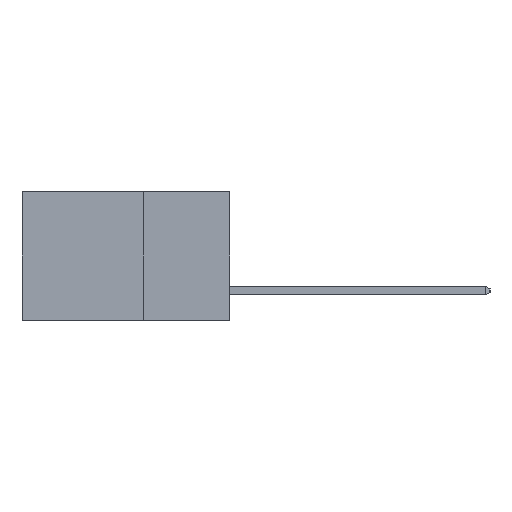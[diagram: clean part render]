
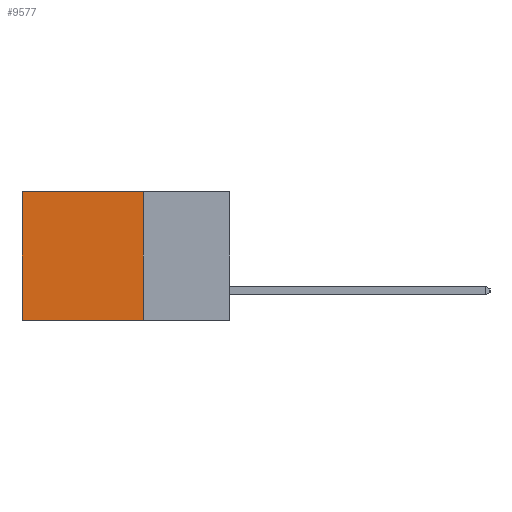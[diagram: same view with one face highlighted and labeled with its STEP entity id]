
A CAD part, left-side view. The second image highlights one B-rep face of the part: STEP entity #9577.
In plain terms, the highlighted planar face has unit normal (-1, 0, 0).
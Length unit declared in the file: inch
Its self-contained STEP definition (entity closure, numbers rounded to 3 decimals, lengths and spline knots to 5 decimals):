
#45 = ORIENTED_EDGE ( 'NONE', *, *, #4189, .F. ) ;
#303 = CARTESIAN_POINT ( 'NONE',  ( 0.298, 0.25, 0. ) ) ;
#1175 = LINE ( 'NONE', #14276, #4788 ) ;
#3883 = AXIS2_PLACEMENT_3D ( 'NONE', #303, #17476, #8109 ) ;
#4189 = EDGE_CURVE ( 'NONE', #13730, #6441, #7310, .T. ) ;
#4197 = ORIENTED_EDGE ( 'NONE', *, *, #18765, .T. ) ;
#4788 = VECTOR ( 'NONE', #6432, 39.37008 ) ;
#4801 = DIRECTION ( 'NONE',  ( 0., 0., -1. ) ) ;
#5476 = VERTEX_POINT ( 'NONE', #19278 ) ;
#5900 = CARTESIAN_POINT ( 'NONE',  ( 0.298, 0.25, -0.37 ) ) ;
#6020 = CARTESIAN_POINT ( 'NONE',  ( 0.298, 0.25, -0.37 ) ) ;
#6432 = DIRECTION ( 'NONE',  ( 0., 1., 0. ) ) ;
#6441 = VERTEX_POINT ( 'NONE', #9092 ) ;
#6531 = PLANE ( 'NONE',  #3883 ) ;
#7228 = VECTOR ( 'NONE', #4801, 39.37008 ) ;
#7310 = LINE ( 'NONE', #6020, #19258 ) ;
#7966 = CARTESIAN_POINT ( 'NONE',  ( 0.298, 0.6, 0. ) ) ;
#8109 = DIRECTION ( 'NONE',  ( 0., 0., -1. ) ) ;
#8846 = EDGE_CURVE ( 'NONE', #15773, #5476, #1175, .T. ) ;
#9083 = ORIENTED_EDGE ( 'NONE', *, *, #10213, .F. ) ;
#9092 = CARTESIAN_POINT ( 'NONE',  ( 0.298, 0.6, -0.37 ) ) ;
#9424 = FACE_OUTER_BOUND ( 'NONE', #10137, .T. ) ;
#9577 = ADVANCED_FACE ( 'NONE', ( #9424 ), #6531, .F. ) ;
#10137 = EDGE_LOOP ( 'NONE', ( #4197, #45, #9083, #14771 ) ) ;
#10213 = EDGE_CURVE ( 'NONE', #15773, #13730, #17963, .T. ) ;
#13082 = DIRECTION ( 'NONE',  ( 0., 0., -1. ) ) ;
#13653 = CARTESIAN_POINT ( 'NONE',  ( 0.298, 0.25, 0. ) ) ;
#13730 = VERTEX_POINT ( 'NONE', #5900 ) ;
#14276 = CARTESIAN_POINT ( 'NONE',  ( 0.298, 0.25, 0. ) ) ;
#14623 = CARTESIAN_POINT ( 'NONE',  ( 0.298, 0.25, 0. ) ) ;
#14771 = ORIENTED_EDGE ( 'NONE', *, *, #8846, .T. ) ;
#15569 = LINE ( 'NONE', #7966, #7228 ) ;
#15773 = VERTEX_POINT ( 'NONE', #13653 ) ;
#17467 = VECTOR ( 'NONE', #13082, 39.37008 ) ;
#17476 = DIRECTION ( 'NONE',  ( 1., 0., 0. ) ) ;
#17963 = LINE ( 'NONE', #14623, #17467 ) ;
#18501 = DIRECTION ( 'NONE',  ( 0., 1., 0. ) ) ;
#18765 = EDGE_CURVE ( 'NONE', #5476, #6441, #15569, .T. ) ;
#19258 = VECTOR ( 'NONE', #18501, 39.37008 ) ;
#19278 = CARTESIAN_POINT ( 'NONE',  ( 0.298, 0.6, 0. ) ) ;
